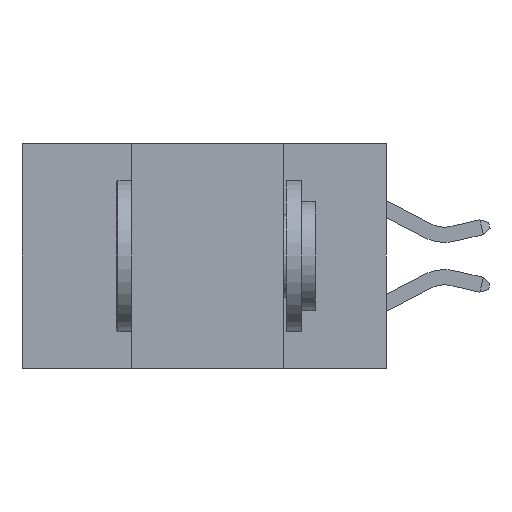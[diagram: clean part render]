
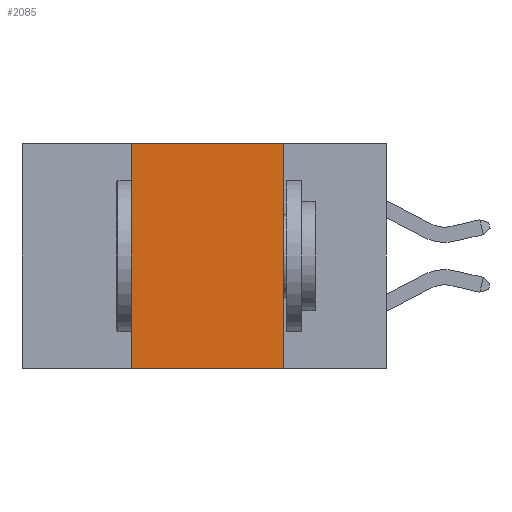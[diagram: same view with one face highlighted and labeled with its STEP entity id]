
A CAD part, left-side view. The second image highlights one B-rep face of the part: STEP entity #2085.
In plain terms, the highlighted planar face has unit normal (-1, 0, 0).
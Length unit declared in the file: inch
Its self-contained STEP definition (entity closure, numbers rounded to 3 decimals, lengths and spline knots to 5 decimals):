
#321 = CARTESIAN_POINT ( 'NONE',  ( 0., 0.42, -0.37 ) ) ;
#708 = ORIENTED_EDGE ( 'NONE', *, *, #14216, .F. ) ;
#1147 = PLANE ( 'NONE',  #16321 ) ;
#1887 = LINE ( 'NONE', #16547, #17038 ) ;
#2085 = ADVANCED_FACE ( 'NONE', ( #8875 ), #1147, .F. ) ;
#2320 = ORIENTED_EDGE ( 'NONE', *, *, #10553, .F. ) ;
#2853 = DIRECTION ( 'NONE',  ( 1., 0., 0. ) ) ;
#3054 = DIRECTION ( 'NONE',  ( 0., 0., 1. ) ) ;
#3242 = VERTEX_POINT ( 'NONE', #9112 ) ;
#3521 = LINE ( 'NONE', #16752, #3981 ) ;
#3981 = VECTOR ( 'NONE', #15029, 39.37008 ) ;
#4335 = ORIENTED_EDGE ( 'NONE', *, *, #9655, .F. ) ;
#4399 = CARTESIAN_POINT ( 'NONE',  ( 0., 0.42, -0.37 ) ) ;
#4920 = VERTEX_POINT ( 'NONE', #321 ) ;
#6777 = CARTESIAN_POINT ( 'NONE',  ( 0., 0.6, -0.37 ) ) ;
#7363 = LINE ( 'NONE', #4399, #12296 ) ;
#7976 = EDGE_LOOP ( 'NONE', ( #4335, #2320, #708, #10724 ) ) ;
#8783 = CARTESIAN_POINT ( 'NONE',  ( 0., 0.6, 0. ) ) ;
#8875 = FACE_OUTER_BOUND ( 'NONE', #7976, .T. ) ;
#9112 = CARTESIAN_POINT ( 'NONE',  ( 0., 0.42, 0. ) ) ;
#9655 = EDGE_CURVE ( 'NONE', #12177, #17878, #1887, .T. ) ;
#10553 = EDGE_CURVE ( 'NONE', #3242, #12177, #3521, .T. ) ;
#10724 = ORIENTED_EDGE ( 'NONE', *, *, #17591, .T. ) ;
#12090 = CARTESIAN_POINT ( 'NONE',  ( 0., 0.17, -0.37 ) ) ;
#12177 = VERTEX_POINT ( 'NONE', #12349 ) ;
#12296 = VECTOR ( 'NONE', #3054, 39.37008 ) ;
#12349 = CARTESIAN_POINT ( 'NONE',  ( 0., 0.17, 0. ) ) ;
#13528 = DIRECTION ( 'NONE',  ( 0., 0., -1. ) ) ;
#14216 = EDGE_CURVE ( 'NONE', #4920, #3242, #7363, .T. ) ;
#15029 = DIRECTION ( 'NONE',  ( 0., -1., 0. ) ) ;
#16321 = AXIS2_PLACEMENT_3D ( 'NONE', #8783, #2853, #17329 ) ;
#16547 = CARTESIAN_POINT ( 'NONE',  ( 0., 0.17, -0.37 ) ) ;
#16752 = CARTESIAN_POINT ( 'NONE',  ( 0., 0.6, 0. ) ) ;
#16764 = LINE ( 'NONE', #6777, #16884 ) ;
#16884 = VECTOR ( 'NONE', #18557, 39.37008 ) ;
#17038 = VECTOR ( 'NONE', #13528, 39.37008 ) ;
#17329 = DIRECTION ( 'NONE',  ( 0., 0., -1. ) ) ;
#17591 = EDGE_CURVE ( 'NONE', #4920, #17878, #16764, .T. ) ;
#17878 = VERTEX_POINT ( 'NONE', #12090 ) ;
#18557 = DIRECTION ( 'NONE',  ( 0., -1., 0. ) ) ;
